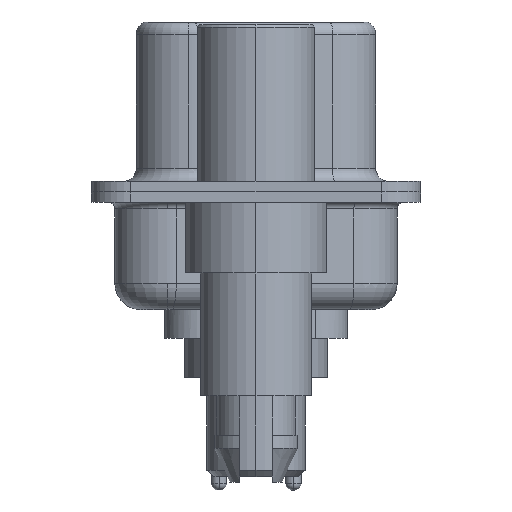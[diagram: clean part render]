
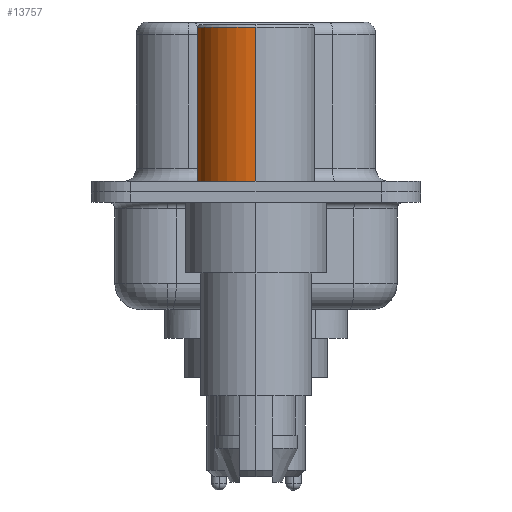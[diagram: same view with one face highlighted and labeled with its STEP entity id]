
A CAD part, left-side view. The second image highlights one B-rep face of the part: STEP entity #13757.
In plain terms, the highlighted cylindrical face has radius 2.25 mm (diameter 4.5 mm), a partial arc.
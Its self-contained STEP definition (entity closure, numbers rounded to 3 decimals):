
#592 = EDGE_LOOP ( 'NONE', ( #13445, #16008, #20206, #20903 ) ) ;
#609 = EDGE_CURVE ( 'NONE', #5554, #1239, #3640, .T. ) ;
#697 = CARTESIAN_POINT ( 'NONE',  ( -2.25, 0., 0.581 ) ) ;
#1239 = VERTEX_POINT ( 'NONE', #14146 ) ;
#3396 = VERTEX_POINT ( 'NONE', #4523 ) ;
#3640 = CIRCLE ( 'NONE', #6555, 2.25 ) ;
#3729 = CARTESIAN_POINT ( 'NONE',  ( 2.25, 0., 0.581 ) ) ;
#4523 = CARTESIAN_POINT ( 'NONE',  ( 2.25, 0., 0.4 ) ) ;
#4752 = LINE ( 'NONE', #697, #22210 ) ;
#5554 = VERTEX_POINT ( 'NONE', #6721 ) ;
#5940 = AXIS2_PLACEMENT_3D ( 'NONE', #20480, #20789, #8309 ) ;
#6555 = AXIS2_PLACEMENT_3D ( 'NONE', #18063, #19912, #12634 ) ;
#6721 = CARTESIAN_POINT ( 'NONE',  ( 2.25, 0., 6.3 ) ) ;
#7947 = DIRECTION ( 'NONE',  ( 1., 0., 0. ) ) ;
#7970 = CIRCLE ( 'NONE', #12348, 2.25 ) ;
#8309 = DIRECTION ( 'NONE',  ( 1., 0., 0. ) ) ;
#9100 = FACE_OUTER_BOUND ( 'NONE', #592, .T. ) ;
#9135 = LINE ( 'NONE', #3729, #14103 ) ;
#10588 = CARTESIAN_POINT ( 'NONE',  ( -2.25, 0., 0.4 ) ) ;
#11458 = DIRECTION ( 'NONE',  ( 0., 0., 1. ) ) ;
#11664 = DIRECTION ( 'NONE',  ( 0., 0., 1. ) ) ;
#12165 = CYLINDRICAL_SURFACE ( 'NONE', #5940, 2.25 ) ;
#12348 = AXIS2_PLACEMENT_3D ( 'NONE', #22046, #11458, #7947 ) ;
#12634 = DIRECTION ( 'NONE',  ( 1., 0., 0. ) ) ;
#13379 = EDGE_CURVE ( 'NONE', #3396, #18119, #7970, .T. ) ;
#13445 = ORIENTED_EDGE ( 'NONE', *, *, #13379, .T. ) ;
#13757 = ADVANCED_FACE ( 'NONE', ( #9100 ), #12165, .T. ) ;
#14103 = VECTOR ( 'NONE', #22892, 1000. ) ;
#14146 = CARTESIAN_POINT ( 'NONE',  ( -2.25, 0., 6.3 ) ) ;
#16008 = ORIENTED_EDGE ( 'NONE', *, *, #21964, .T. ) ;
#18063 = CARTESIAN_POINT ( 'NONE',  ( 0., 0., 6.3 ) ) ;
#18119 = VERTEX_POINT ( 'NONE', #10588 ) ;
#19069 = EDGE_CURVE ( 'NONE', #3396, #5554, #9135, .T. ) ;
#19912 = DIRECTION ( 'NONE',  ( 0., 0., 1. ) ) ;
#20206 = ORIENTED_EDGE ( 'NONE', *, *, #609, .F. ) ;
#20480 = CARTESIAN_POINT ( 'NONE',  ( 0., 0., 0.581 ) ) ;
#20789 = DIRECTION ( 'NONE',  ( 0., 0., 1. ) ) ;
#20903 = ORIENTED_EDGE ( 'NONE', *, *, #19069, .F. ) ;
#21964 = EDGE_CURVE ( 'NONE', #18119, #1239, #4752, .T. ) ;
#22046 = CARTESIAN_POINT ( 'NONE',  ( 0., 0., 0.4 ) ) ;
#22210 = VECTOR ( 'NONE', #11664, 1000. ) ;
#22892 = DIRECTION ( 'NONE',  ( 0., 0., 1. ) ) ;
